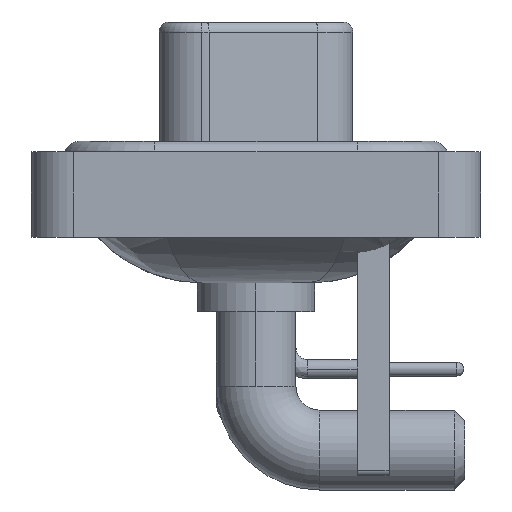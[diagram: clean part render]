
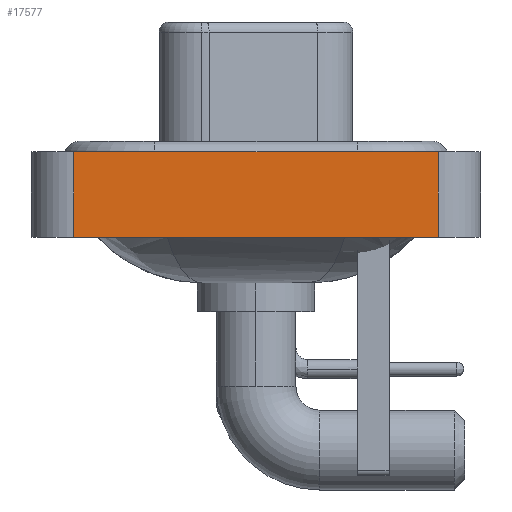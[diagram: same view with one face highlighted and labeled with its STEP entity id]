
A CAD part, left-side view. The second image highlights one B-rep face of the part: STEP entity #17577.
In plain terms, the highlighted planar face has unit normal (-1, 0, 0).
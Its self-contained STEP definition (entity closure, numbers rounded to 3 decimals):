
#1468 = VERTEX_POINT ( 'NONE', #15533 ) ;
#1777 = ORIENTED_EDGE ( 'NONE', *, *, #20152, .F. ) ;
#1888 = VERTEX_POINT ( 'NONE', #19935 ) ;
#3208 = LINE ( 'NONE', #25637, #5549 ) ;
#3483 = EDGE_CURVE ( 'NONE', #4878, #1468, #18825, .T. ) ;
#4043 = ORIENTED_EDGE ( 'NONE', *, *, #22781, .T. ) ;
#4252 = CARTESIAN_POINT ( 'NONE',  ( -7.35, -8.55, -3.6 ) ) ;
#4878 = VERTEX_POINT ( 'NONE', #4252 ) ;
#5549 = VECTOR ( 'NONE', #7037, 1000. ) ;
#5800 = CARTESIAN_POINT ( 'NONE',  ( -7.35, -8.55, 0.4 ) ) ;
#6380 = VECTOR ( 'NONE', #22352, 1000. ) ;
#6436 = PLANE ( 'NONE',  #10141 ) ;
#6909 = EDGE_LOOP ( 'NONE', ( #26572, #17563, #1777, #4043 ) ) ;
#7037 = DIRECTION ( 'NONE',  ( 0., -1., 0. ) ) ;
#7079 = FACE_OUTER_BOUND ( 'NONE', #6909, .T. ) ;
#7157 = VECTOR ( 'NONE', #17170, 1000. ) ;
#7211 = CARTESIAN_POINT ( 'NONE',  ( -7.35, -8.55, -3.6 ) ) ;
#8096 = LINE ( 'NONE', #5800, #6380 ) ;
#8905 = CARTESIAN_POINT ( 'NONE',  ( -7.35, 8.55, -3.6 ) ) ;
#9682 = EDGE_CURVE ( 'NONE', #1888, #1468, #8096, .T. ) ;
#10141 = AXIS2_PLACEMENT_3D ( 'NONE', #7211, #14584, #10649 ) ;
#10649 = DIRECTION ( 'NONE',  ( 0., 0., 1. ) ) ;
#11110 = VERTEX_POINT ( 'NONE', #15175 ) ;
#14584 = DIRECTION ( 'NONE',  ( -1., 0., 0. ) ) ;
#14896 = DIRECTION ( 'NONE',  ( 0., 0., 1. ) ) ;
#15175 = CARTESIAN_POINT ( 'NONE',  ( -7.35, 8.55, -3.6 ) ) ;
#15533 = CARTESIAN_POINT ( 'NONE',  ( -7.35, -8.55, 0.4 ) ) ;
#17170 = DIRECTION ( 'NONE',  ( 0., 0., 1. ) ) ;
#17304 = LINE ( 'NONE', #8905, #7157 ) ;
#17563 = ORIENTED_EDGE ( 'NONE', *, *, #9682, .F. ) ;
#17577 = ADVANCED_FACE ( 'NONE', ( #7079 ), #6436, .T. ) ;
#18825 = LINE ( 'NONE', #25218, #24340 ) ;
#19935 = CARTESIAN_POINT ( 'NONE',  ( -7.35, 8.55, 0.4 ) ) ;
#20152 = EDGE_CURVE ( 'NONE', #11110, #1888, #17304, .T. ) ;
#22352 = DIRECTION ( 'NONE',  ( 0., -1., 0. ) ) ;
#22781 = EDGE_CURVE ( 'NONE', #11110, #4878, #3208, .T. ) ;
#24340 = VECTOR ( 'NONE', #14896, 1000. ) ;
#25218 = CARTESIAN_POINT ( 'NONE',  ( -7.35, -8.55, -3.6 ) ) ;
#25637 = CARTESIAN_POINT ( 'NONE',  ( -7.35, -8.55, -3.6 ) ) ;
#26572 = ORIENTED_EDGE ( 'NONE', *, *, #3483, .T. ) ;
